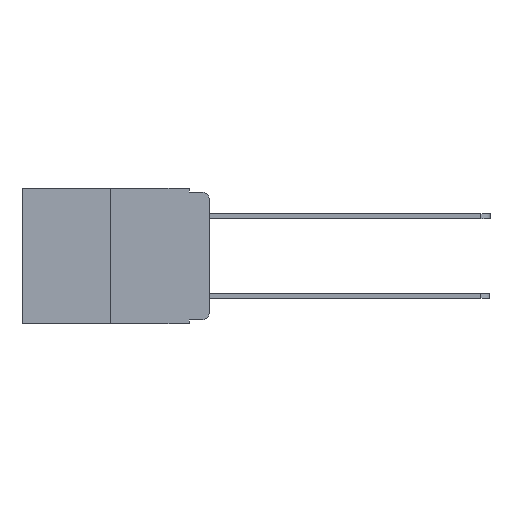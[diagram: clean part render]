
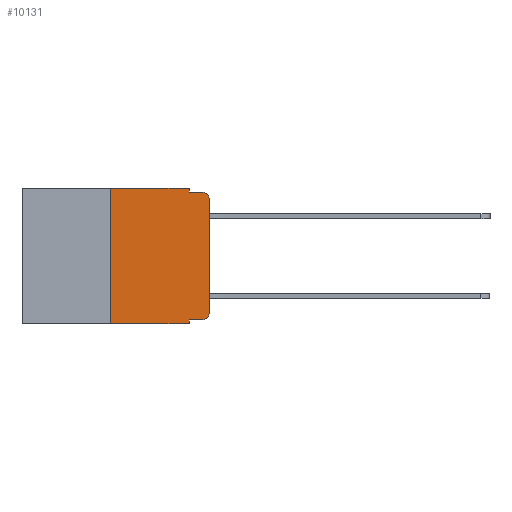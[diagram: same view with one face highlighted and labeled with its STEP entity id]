
A CAD part, left-side view. The second image highlights one B-rep face of the part: STEP entity #10131.
In plain terms, the highlighted planar face has unit normal (-1, 0, 0).
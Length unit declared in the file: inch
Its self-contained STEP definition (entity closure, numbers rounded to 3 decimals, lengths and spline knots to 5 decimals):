
#56 = DIRECTION ( 'NONE',  ( 0., 0., -1. ) ) ;
#177 = ORIENTED_EDGE ( 'NONE', *, *, #18067, .T. ) ;
#506 = CARTESIAN_POINT ( 'NONE',  ( 0., 0., -0.313 ) ) ;
#965 = ORIENTED_EDGE ( 'NONE', *, *, #19149, .T. ) ;
#1713 = CARTESIAN_POINT ( 'NONE',  ( 0., 0.051, 0. ) ) ;
#2001 = CIRCLE ( 'NONE', #18953, 0.02 ) ;
#2032 = DIRECTION ( 'NONE',  ( 1., 0., 0. ) ) ;
#2273 = ORIENTED_EDGE ( 'NONE', *, *, #12474, .F. ) ;
#2300 = ORIENTED_EDGE ( 'NONE', *, *, #16114, .F. ) ;
#2752 = VERTEX_POINT ( 'NONE', #20307 ) ;
#2786 = LINE ( 'NONE', #17509, #7020 ) ;
#2858 = LINE ( 'NONE', #11649, #19608 ) ;
#2863 = LINE ( 'NONE', #1713, #11402 ) ;
#3754 = DIRECTION ( 'NONE',  ( 0., -1., 0. ) ) ;
#3830 = EDGE_CURVE ( 'NONE', #16351, #5004, #2001, .T. ) ;
#3896 = VERTEX_POINT ( 'NONE', #13427 ) ;
#4825 = ORIENTED_EDGE ( 'NONE', *, *, #13180, .T. ) ;
#5004 = VERTEX_POINT ( 'NONE', #506 ) ;
#5083 = EDGE_CURVE ( 'NONE', #2752, #3896, #2786, .T. ) ;
#5213 = VERTEX_POINT ( 'NONE', #6746 ) ;
#5344 = CARTESIAN_POINT ( 'NONE',  ( 0., 0.473, -0.343 ) ) ;
#5513 = VECTOR ( 'NONE', #12635, 39.37008 ) ;
#6325 = EDGE_LOOP ( 'NONE', ( #965, #177, #2300, #2273, #7758, #16895, #17642, #11331, #4825, #19091 ) ) ;
#6667 = EDGE_CURVE ( 'NONE', #5213, #17604, #19678, .T. ) ;
#6746 = CARTESIAN_POINT ( 'NONE',  ( 0., 0.25, 0. ) ) ;
#6747 = LINE ( 'NONE', #20393, #10888 ) ;
#6790 = CARTESIAN_POINT ( 'NONE',  ( 0., 0.02, -0.313 ) ) ;
#7020 = VECTOR ( 'NONE', #9725, 39.37008 ) ;
#7735 = CIRCLE ( 'NONE', #15182, 0.02 ) ;
#7758 = ORIENTED_EDGE ( 'NONE', *, *, #6667, .F. ) ;
#7826 = EDGE_CURVE ( 'NONE', #12872, #5213, #2858, .T. ) ;
#8470 = DIRECTION ( 'NONE',  ( 0., 0., -1. ) ) ;
#8840 = FACE_OUTER_BOUND ( 'NONE', #6325, .T. ) ;
#9001 = VECTOR ( 'NONE', #13513, 39.37008 ) ;
#9725 = DIRECTION ( 'NONE',  ( 0., 0., -1. ) ) ;
#10131 = ADVANCED_FACE ( 'NONE', ( #8840 ), #12207, .F. ) ;
#10186 = DIRECTION ( 'NONE',  ( 0., -1., 0. ) ) ;
#10636 = DIRECTION ( 'NONE',  ( -1., 0., 0. ) ) ;
#10888 = VECTOR ( 'NONE', #11207, 39.37008 ) ;
#11054 = VERTEX_POINT ( 'NONE', #15719 ) ;
#11207 = DIRECTION ( 'NONE',  ( 0., 0., 1. ) ) ;
#11331 = ORIENTED_EDGE ( 'NONE', *, *, #5083, .F. ) ;
#11402 = VECTOR ( 'NONE', #19702, 39.37008 ) ;
#11649 = CARTESIAN_POINT ( 'NONE',  ( 0., 0.25, 0. ) ) ;
#11767 = CARTESIAN_POINT ( 'NONE',  ( 0., 0.051, -0.01 ) ) ;
#11885 = CARTESIAN_POINT ( 'NONE',  ( 0., 0.051, 0. ) ) ;
#12207 = PLANE ( 'NONE',  #18187 ) ;
#12474 = EDGE_CURVE ( 'NONE', #17604, #18607, #2863, .T. ) ;
#12635 = DIRECTION ( 'NONE',  ( 0., -1., 0. ) ) ;
#12872 = VERTEX_POINT ( 'NONE', #14597 ) ;
#13164 = LINE ( 'NONE', #5344, #9001 ) ;
#13177 = DIRECTION ( 'NONE',  ( 0., 0., 1. ) ) ;
#13180 = EDGE_CURVE ( 'NONE', #2752, #16351, #17713, .T. ) ;
#13427 = CARTESIAN_POINT ( 'NONE',  ( 0., 0.051, -0.343 ) ) ;
#13513 = DIRECTION ( 'NONE',  ( 0., -1., 0. ) ) ;
#13649 = CARTESIAN_POINT ( 'NONE',  ( 0., 0.051, -0.333 ) ) ;
#13755 = DIRECTION ( 'NONE',  ( 0., 0., -1. ) ) ;
#13797 = CARTESIAN_POINT ( 'NONE',  ( 0., 0.02, -0.333 ) ) ;
#14492 = VERTEX_POINT ( 'NONE', #16076 ) ;
#14597 = CARTESIAN_POINT ( 'NONE',  ( 0., 0.25, -0.343 ) ) ;
#15182 = AXIS2_PLACEMENT_3D ( 'NONE', #19862, #10636, #56 ) ;
#15719 = CARTESIAN_POINT ( 'NONE',  ( 0., 0., -0.03 ) ) ;
#16076 = CARTESIAN_POINT ( 'NONE',  ( 0., 0.02, -0.01 ) ) ;
#16114 = EDGE_CURVE ( 'NONE', #18607, #14492, #17615, .T. ) ;
#16258 = CARTESIAN_POINT ( 'NONE',  ( 0., 0.051, -0.01 ) ) ;
#16351 = VERTEX_POINT ( 'NONE', #13797 ) ;
#16895 = ORIENTED_EDGE ( 'NONE', *, *, #7826, .F. ) ;
#16923 = EDGE_CURVE ( 'NONE', #12872, #3896, #13164, .T. ) ;
#17146 = VECTOR ( 'NONE', #10186, 39.37008 ) ;
#17509 = CARTESIAN_POINT ( 'NONE',  ( 0., 0.051, 0. ) ) ;
#17604 = VERTEX_POINT ( 'NONE', #11885 ) ;
#17615 = LINE ( 'NONE', #11767, #17146 ) ;
#17642 = ORIENTED_EDGE ( 'NONE', *, *, #16923, .T. ) ;
#17713 = LINE ( 'NONE', #13649, #21166 ) ;
#17875 = DIRECTION ( 'NONE',  ( -1., 0., 0. ) ) ;
#18067 = EDGE_CURVE ( 'NONE', #11054, #14492, #7735, .T. ) ;
#18187 = AXIS2_PLACEMENT_3D ( 'NONE', #19892, #2032, #13755 ) ;
#18607 = VERTEX_POINT ( 'NONE', #16258 ) ;
#18820 = CARTESIAN_POINT ( 'NONE',  ( 0., 0.473, 0. ) ) ;
#18953 = AXIS2_PLACEMENT_3D ( 'NONE', #6790, #17875, #8470 ) ;
#19091 = ORIENTED_EDGE ( 'NONE', *, *, #3830, .T. ) ;
#19149 = EDGE_CURVE ( 'NONE', #5004, #11054, #6747, .T. ) ;
#19608 = VECTOR ( 'NONE', #13177, 39.37008 ) ;
#19678 = LINE ( 'NONE', #18820, #5513 ) ;
#19702 = DIRECTION ( 'NONE',  ( 0., 0., -1. ) ) ;
#19862 = CARTESIAN_POINT ( 'NONE',  ( 0., 0.02, -0.03 ) ) ;
#19892 = CARTESIAN_POINT ( 'NONE',  ( 0., 0.473, 0. ) ) ;
#20307 = CARTESIAN_POINT ( 'NONE',  ( 0., 0.051, -0.333 ) ) ;
#20393 = CARTESIAN_POINT ( 'NONE',  ( 0., 0., 0. ) ) ;
#21166 = VECTOR ( 'NONE', #3754, 39.37008 ) ;
